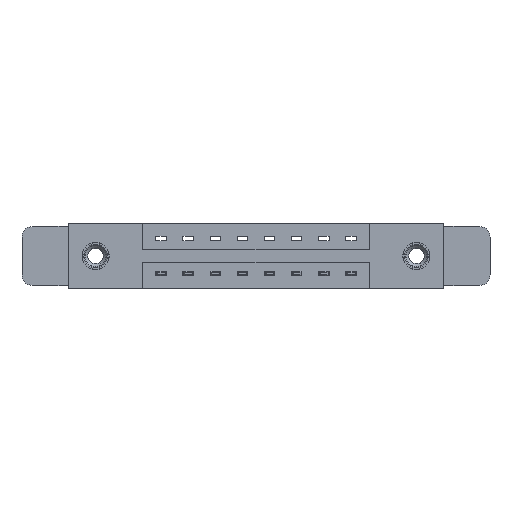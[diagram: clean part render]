
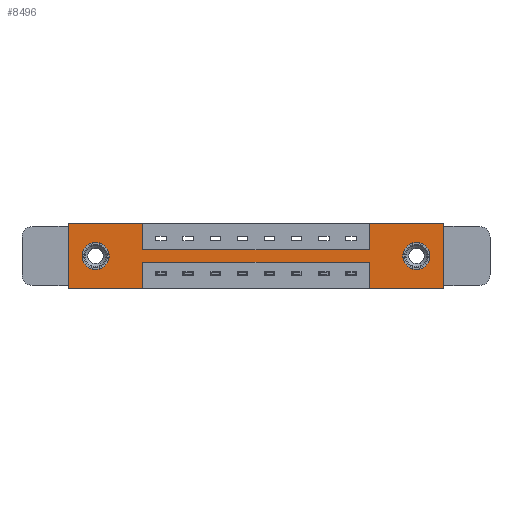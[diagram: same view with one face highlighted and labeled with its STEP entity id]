
A CAD part, front view. The second image highlights one B-rep face of the part: STEP entity #8496.
In plain terms, the highlighted planar face has unit normal (0, -1, 0).
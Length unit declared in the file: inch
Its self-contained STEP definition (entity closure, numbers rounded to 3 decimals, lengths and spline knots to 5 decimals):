
#226 = DIRECTION ( 'NONE',  ( 0., 0., 1. ) ) ;
#343 = DIRECTION ( 'NONE',  ( 0., 0., 1. ) ) ;
#362 = VERTEX_POINT ( 'NONE', #2998 ) ;
#511 = CIRCLE ( 'NONE', #7487, 0.078 ) ;
#545 = ORIENTED_EDGE ( 'NONE', *, *, #11658, .F. ) ;
#589 = ORIENTED_EDGE ( 'NONE', *, *, #7271, .F. ) ;
#613 = CARTESIAN_POINT ( 'NONE',  ( 0.155, 0., -0.185 ) ) ;
#678 = VERTEX_POINT ( 'NONE', #3241 ) ;
#769 = VERTEX_POINT ( 'NONE', #5661 ) ;
#793 = CIRCLE ( 'NONE', #7631, 0.078 ) ;
#823 = EDGE_LOOP ( 'NONE', ( #7753, #12228 ) ) ;
#877 = CARTESIAN_POINT ( 'NONE',  ( 1.729, 0., -0.37 ) ) ;
#951 = CARTESIAN_POINT ( 'NONE',  ( 0.425, 0., -0.15 ) ) ;
#992 = VECTOR ( 'NONE', #10189, 39.37008 ) ;
#1048 = EDGE_CURVE ( 'NONE', #769, #10152, #3756, .T. ) ;
#1464 = LINE ( 'NONE', #10626, #5689 ) ;
#1565 = ORIENTED_EDGE ( 'NONE', *, *, #5254, .F. ) ;
#1614 = VERTEX_POINT ( 'NONE', #12192 ) ;
#1660 = DIRECTION ( 'NONE',  ( -1., 0., 0. ) ) ;
#1700 = EDGE_CURVE ( 'NONE', #1754, #10293, #12516, .T. ) ;
#1754 = VERTEX_POINT ( 'NONE', #2636 ) ;
#1904 = VECTOR ( 'NONE', #12074, 39.37008 ) ;
#2047 = AXIS2_PLACEMENT_3D ( 'NONE', #10342, #7276, #2321 ) ;
#2092 = DIRECTION ( 'NONE',  ( -1., 0., 0. ) ) ;
#2201 = VECTOR ( 'NONE', #343, 39.37008 ) ;
#2244 = DIRECTION ( 'NONE',  ( 0., 0., -1. ) ) ;
#2278 = CARTESIAN_POINT ( 'NONE',  ( 0.425, 0., -0.15 ) ) ;
#2321 = DIRECTION ( 'NONE',  ( 0., 0., -1. ) ) ;
#2331 = CARTESIAN_POINT ( 'NONE',  ( 1.729, 0., 0. ) ) ;
#2386 = VECTOR ( 'NONE', #226, 39.37008 ) ;
#2416 = DIRECTION ( 'NONE',  ( 1., 0., 0. ) ) ;
#2417 = VERTEX_POINT ( 'NONE', #11941 ) ;
#2445 = LINE ( 'NONE', #2278, #9591 ) ;
#2602 = EDGE_LOOP ( 'NONE', ( #8023, #9327 ) ) ;
#2636 = CARTESIAN_POINT ( 'NONE',  ( 0., 0., 0. ) ) ;
#2938 = ORIENTED_EDGE ( 'NONE', *, *, #8334, .F. ) ;
#2998 = CARTESIAN_POINT ( 'NONE',  ( 0.155, 0., -0.107 ) ) ;
#3076 = CARTESIAN_POINT ( 'NONE',  ( 0.425, 0., -0.22 ) ) ;
#3116 = AXIS2_PLACEMENT_3D ( 'NONE', #613, #12491, #4509 ) ;
#3215 = DIRECTION ( 'NONE',  ( 0., 0., -1. ) ) ;
#3241 = CARTESIAN_POINT ( 'NONE',  ( 0.425, 0., -0.37 ) ) ;
#3306 = PLANE ( 'NONE',  #2047 ) ;
#3492 = ORIENTED_EDGE ( 'NONE', *, *, #5154, .F. ) ;
#3551 = VECTOR ( 'NONE', #2092, 39.37008 ) ;
#3667 = LINE ( 'NONE', #4292, #7690 ) ;
#3756 = LINE ( 'NONE', #3811, #11303 ) ;
#3811 = CARTESIAN_POINT ( 'NONE',  ( 0., 0., -0.37 ) ) ;
#3904 = EDGE_CURVE ( 'NONE', #10854, #362, #9557, .T. ) ;
#4292 = CARTESIAN_POINT ( 'NONE',  ( 0.425, 0., 0. ) ) ;
#4509 = DIRECTION ( 'NONE',  ( 0., 0., 1. ) ) ;
#4750 = LINE ( 'NONE', #10980, #2386 ) ;
#5004 = VERTEX_POINT ( 'NONE', #11965 ) ;
#5071 = DIRECTION ( 'NONE',  ( 0., 1., 0. ) ) ;
#5105 = ORIENTED_EDGE ( 'NONE', *, *, #1048, .F. ) ;
#5154 = EDGE_CURVE ( 'NONE', #5965, #678, #11337, .T. ) ;
#5230 = DIRECTION ( 'NONE',  ( 0., 1., 0. ) ) ;
#5254 = EDGE_CURVE ( 'NONE', #2417, #10128, #9522, .T. ) ;
#5266 = DIRECTION ( 'NONE',  ( 0., 1., 0. ) ) ;
#5661 = CARTESIAN_POINT ( 'NONE',  ( 2.154, 0., -0.37 ) ) ;
#5667 = VERTEX_POINT ( 'NONE', #7397 ) ;
#5671 = CIRCLE ( 'NONE', #10015, 0.078 ) ;
#5689 = VECTOR ( 'NONE', #2416, 39.37008 ) ;
#5761 = CARTESIAN_POINT ( 'NONE',  ( 0.155, 0., -0.263 ) ) ;
#5792 = EDGE_CURVE ( 'NONE', #10152, #6234, #9043, .T. ) ;
#5877 = CARTESIAN_POINT ( 'NONE',  ( 1.729, 0., -0.22 ) ) ;
#5965 = VERTEX_POINT ( 'NONE', #12670 ) ;
#6083 = ORIENTED_EDGE ( 'NONE', *, *, #9800, .F. ) ;
#6234 = VERTEX_POINT ( 'NONE', #5877 ) ;
#6267 = VECTOR ( 'NONE', #11237, 39.37008 ) ;
#6298 = CARTESIAN_POINT ( 'NONE',  ( 2.154, 0., 0. ) ) ;
#6420 = ORIENTED_EDGE ( 'NONE', *, *, #12049, .F. ) ;
#6543 = ORIENTED_EDGE ( 'NONE', *, *, #5792, .F. ) ;
#6684 = EDGE_CURVE ( 'NONE', #362, #10854, #5671, .T. ) ;
#6774 = CARTESIAN_POINT ( 'NONE',  ( 0., 0., -0.37 ) ) ;
#6879 = CARTESIAN_POINT ( 'NONE',  ( 0.155, 0., -0.185 ) ) ;
#6882 = ORIENTED_EDGE ( 'NONE', *, *, #1700, .F. ) ;
#7098 = CARTESIAN_POINT ( 'NONE',  ( 0.425, 0., -0.37 ) ) ;
#7101 = LINE ( 'NONE', #3076, #3551 ) ;
#7181 = VECTOR ( 'NONE', #10559, 39.37008 ) ;
#7271 = EDGE_CURVE ( 'NONE', #5667, #769, #10758, .T. ) ;
#7276 = DIRECTION ( 'NONE',  ( 0., -1., 0. ) ) ;
#7397 = CARTESIAN_POINT ( 'NONE',  ( 2.154, 0., 0. ) ) ;
#7487 = AXIS2_PLACEMENT_3D ( 'NONE', #11113, #5266, #12137 ) ;
#7631 = AXIS2_PLACEMENT_3D ( 'NONE', #10190, #5230, #2244 ) ;
#7690 = VECTOR ( 'NONE', #3215, 39.37008 ) ;
#7753 = ORIENTED_EDGE ( 'NONE', *, *, #8723, .T. ) ;
#7790 = VECTOR ( 'NONE', #12191, 39.37008 ) ;
#7982 = DIRECTION ( 'NONE',  ( 0., 0., 1. ) ) ;
#8023 = ORIENTED_EDGE ( 'NONE', *, *, #6684, .T. ) ;
#8212 = DIRECTION ( 'NONE',  ( 1., 0., 0. ) ) ;
#8334 = EDGE_CURVE ( 'NONE', #678, #5004, #12382, .T. ) ;
#8496 = ADVANCED_FACE ( 'NONE', ( #11783, #9194, #12256 ), #3306, .T. ) ;
#8704 = CARTESIAN_POINT ( 'NONE',  ( 1.999, 0., -0.263 ) ) ;
#8723 = EDGE_CURVE ( 'NONE', #1614, #11614, #793, .T. ) ;
#8797 = CARTESIAN_POINT ( 'NONE',  ( 1.729, 0., 0. ) ) ;
#9043 = LINE ( 'NONE', #9382, #2201 ) ;
#9194 = FACE_BOUND ( 'NONE', #2602, .T. ) ;
#9249 = CARTESIAN_POINT ( 'NONE',  ( 0., 0., 0. ) ) ;
#9327 = ORIENTED_EDGE ( 'NONE', *, *, #3904, .T. ) ;
#9382 = CARTESIAN_POINT ( 'NONE',  ( 1.729, 0., -0.37 ) ) ;
#9522 = LINE ( 'NONE', #2331, #6267 ) ;
#9557 = CIRCLE ( 'NONE', #3116, 0.078 ) ;
#9591 = VECTOR ( 'NONE', #8212, 39.37008 ) ;
#9800 = EDGE_CURVE ( 'NONE', #11035, #2417, #2445, .T. ) ;
#10015 = AXIS2_PLACEMENT_3D ( 'NONE', #6879, #5071, #7982 ) ;
#10128 = VERTEX_POINT ( 'NONE', #8797 ) ;
#10152 = VERTEX_POINT ( 'NONE', #877 ) ;
#10189 = DIRECTION ( 'NONE',  ( 0., 0., -1. ) ) ;
#10190 = CARTESIAN_POINT ( 'NONE',  ( 1.999, 0., -0.185 ) ) ;
#10284 = EDGE_CURVE ( 'NONE', #6234, #5965, #7101, .T. ) ;
#10293 = VERTEX_POINT ( 'NONE', #12019 ) ;
#10342 = CARTESIAN_POINT ( 'NONE',  ( 0., 0., -0.37 ) ) ;
#10559 = DIRECTION ( 'NONE',  ( -1., 0., 0. ) ) ;
#10626 = CARTESIAN_POINT ( 'NONE',  ( 0., 0., 0. ) ) ;
#10758 = LINE ( 'NONE', #6298, #992 ) ;
#10854 = VERTEX_POINT ( 'NONE', #5761 ) ;
#10980 = CARTESIAN_POINT ( 'NONE',  ( 0., 0., 0. ) ) ;
#11035 = VERTEX_POINT ( 'NONE', #951 ) ;
#11113 = CARTESIAN_POINT ( 'NONE',  ( 1.999, 0., -0.185 ) ) ;
#11237 = DIRECTION ( 'NONE',  ( 0., 0., 1. ) ) ;
#11303 = VECTOR ( 'NONE', #1660, 39.37008 ) ;
#11337 = LINE ( 'NONE', #7098, #1904 ) ;
#11365 = ORIENTED_EDGE ( 'NONE', *, *, #12568, .F. ) ;
#11614 = VERTEX_POINT ( 'NONE', #8704 ) ;
#11621 = ORIENTED_EDGE ( 'NONE', *, *, #10284, .F. ) ;
#11658 = EDGE_CURVE ( 'NONE', #10128, #5667, #1464, .T. ) ;
#11783 = FACE_BOUND ( 'NONE', #823, .T. ) ;
#11941 = CARTESIAN_POINT ( 'NONE',  ( 1.729, 0., -0.15 ) ) ;
#11965 = CARTESIAN_POINT ( 'NONE',  ( 0., 0., -0.37 ) ) ;
#12019 = CARTESIAN_POINT ( 'NONE',  ( 0.425, 0., 0. ) ) ;
#12049 = EDGE_CURVE ( 'NONE', #5004, #1754, #4750, .T. ) ;
#12074 = DIRECTION ( 'NONE',  ( 0., 0., -1. ) ) ;
#12119 = EDGE_LOOP ( 'NONE', ( #3492, #11621, #6543, #5105, #589, #545, #1565, #6083, #11365, #6882, #6420, #2938 ) ) ;
#12137 = DIRECTION ( 'NONE',  ( 0., 0., -1. ) ) ;
#12191 = DIRECTION ( 'NONE',  ( 1., 0., 0. ) ) ;
#12192 = CARTESIAN_POINT ( 'NONE',  ( 1.999, 0., -0.107 ) ) ;
#12228 = ORIENTED_EDGE ( 'NONE', *, *, #12777, .T. ) ;
#12256 = FACE_OUTER_BOUND ( 'NONE', #12119, .T. ) ;
#12382 = LINE ( 'NONE', #6774, #7181 ) ;
#12491 = DIRECTION ( 'NONE',  ( 0., 1., 0. ) ) ;
#12516 = LINE ( 'NONE', #9249, #7790 ) ;
#12568 = EDGE_CURVE ( 'NONE', #10293, #11035, #3667, .T. ) ;
#12670 = CARTESIAN_POINT ( 'NONE',  ( 0.425, 0., -0.22 ) ) ;
#12777 = EDGE_CURVE ( 'NONE', #11614, #1614, #511, .T. ) ;
